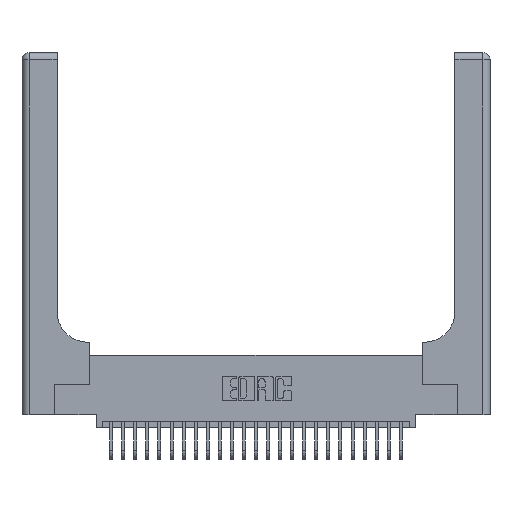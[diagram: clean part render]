
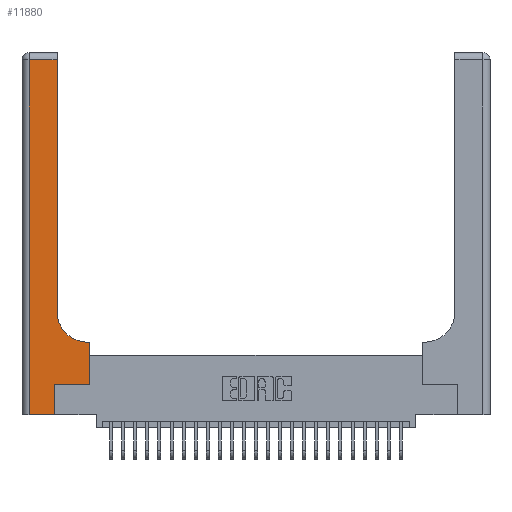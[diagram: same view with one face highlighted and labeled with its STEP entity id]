
A CAD part, top view. The second image highlights one B-rep face of the part: STEP entity #11880.
In plain terms, the highlighted planar face has unit normal (0, 0, 1).
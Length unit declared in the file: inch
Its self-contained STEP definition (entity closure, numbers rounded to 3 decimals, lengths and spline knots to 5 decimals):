
#184 = LINE ( 'NONE', #10783, #22507 ) ;
#234 = VERTEX_POINT ( 'NONE', #27878 ) ;
#263 = LINE ( 'NONE', #14552, #23274 ) ;
#578 = CARTESIAN_POINT ( 'NONE',  ( 0.2915, 2.94, 0.37 ) ) ;
#586 = LINE ( 'NONE', #12785, #11682 ) ;
#957 = VERTEX_POINT ( 'NONE', #14197 ) ;
#1566 = ORIENTED_EDGE ( 'NONE', *, *, #22909, .T. ) ;
#1987 = DIRECTION ( 'NONE',  ( -1., 0., 0. ) ) ;
#2071 = VECTOR ( 'NONE', #10237, 39.37008 ) ;
#2457 = EDGE_CURVE ( 'NONE', #8559, #4400, #23183, .T. ) ;
#3621 = ORIENTED_EDGE ( 'NONE', *, *, #8796, .T. ) ;
#3744 = ORIENTED_EDGE ( 'NONE', *, *, #2457, .T. ) ;
#4316 = EDGE_LOOP ( 'NONE', ( #9998, #3744, #8403, #5873, #7416, #1566, #3621, #21140, #25136 ) ) ;
#4400 = VERTEX_POINT ( 'NONE', #11769 ) ;
#5567 = CARTESIAN_POINT ( 'NONE',  ( 0.5415, 0.85, 0.37 ) ) ;
#5576 = CARTESIAN_POINT ( 'NONE',  ( 0.269, 0., 0.37 ) ) ;
#5873 = ORIENTED_EDGE ( 'NONE', *, *, #6956, .T. ) ;
#5915 = DIRECTION ( 'NONE',  ( 0., 1., 0. ) ) ;
#6107 = VECTOR ( 'NONE', #19537, 39.37008 ) ;
#6956 = EDGE_CURVE ( 'NONE', #22199, #957, #263, .T. ) ;
#7341 = DIRECTION ( 'NONE',  ( 0., 0., -1. ) ) ;
#7416 = ORIENTED_EDGE ( 'NONE', *, *, #25411, .T. ) ;
#7780 = DIRECTION ( 'NONE',  ( 1., 0., 0. ) ) ;
#7938 = DIRECTION ( 'NONE',  ( 1., 0., 0. ) ) ;
#8122 = CARTESIAN_POINT ( 'NONE',  ( 0., 2.94, 0.37 ) ) ;
#8403 = ORIENTED_EDGE ( 'NONE', *, *, #11023, .T. ) ;
#8559 = VERTEX_POINT ( 'NONE', #578 ) ;
#8796 = EDGE_CURVE ( 'NONE', #12746, #11222, #11831, .T. ) ;
#9263 = LINE ( 'NONE', #5576, #14498 ) ;
#9995 = DIRECTION ( 'NONE',  ( 0., 1., 0. ) ) ;
#9998 = ORIENTED_EDGE ( 'NONE', *, *, #26232, .T. ) ;
#10237 = DIRECTION ( 'NONE',  ( 1., 0., 0. ) ) ;
#10783 = CARTESIAN_POINT ( 'NONE',  ( 0.2915, 0.6, 0.37 ) ) ;
#11023 = EDGE_CURVE ( 'NONE', #4400, #22199, #586, .T. ) ;
#11222 = VERTEX_POINT ( 'NONE', #22989 ) ;
#11680 = PLANE ( 'NONE',  #18655 ) ;
#11682 = VECTOR ( 'NONE', #28460, 39.37008 ) ;
#11769 = CARTESIAN_POINT ( 'NONE',  ( 0.06, 2.94, 0.37 ) ) ;
#11831 = LINE ( 'NONE', #14741, #22335 ) ;
#11880 = ADVANCED_FACE ( 'NONE', ( #15141 ), #11680, .F. ) ;
#12746 = VERTEX_POINT ( 'NONE', #25901 ) ;
#12785 = CARTESIAN_POINT ( 'NONE',  ( 0.06, 3., 0.37 ) ) ;
#13308 = CARTESIAN_POINT ( 'NONE',  ( 0.06, 0., 0.37 ) ) ;
#14197 = CARTESIAN_POINT ( 'NONE',  ( 0.269, 0., 0.37 ) ) ;
#14228 = VERTEX_POINT ( 'NONE', #17385 ) ;
#14498 = VECTOR ( 'NONE', #9995, 39.37008 ) ;
#14552 = CARTESIAN_POINT ( 'NONE',  ( 0., 0., 0.37 ) ) ;
#14738 = CARTESIAN_POINT ( 'NONE',  ( 0.5415, 0.6, 0.37 ) ) ;
#14741 = CARTESIAN_POINT ( 'NONE',  ( 0.5585, 0.25, 0.37 ) ) ;
#15045 = CARTESIAN_POINT ( 'NONE',  ( 0.2915, 3., 0.37 ) ) ;
#15141 = FACE_OUTER_BOUND ( 'NONE', #4316, .T. ) ;
#15815 = VERTEX_POINT ( 'NONE', #14738 ) ;
#16176 = CARTESIAN_POINT ( 'NONE',  ( 0., 3., 0.37 ) ) ;
#17213 = VECTOR ( 'NONE', #19243, 39.37008 ) ;
#17385 = CARTESIAN_POINT ( 'NONE',  ( 0.2915, 0.85, 0.37 ) ) ;
#18655 = AXIS2_PLACEMENT_3D ( 'NONE', #16176, #7341, #22952 ) ;
#19243 = DIRECTION ( 'NONE',  ( -1., 0., 0. ) ) ;
#19537 = DIRECTION ( 'NONE',  ( 0., 1., 0. ) ) ;
#20847 = EDGE_CURVE ( 'NONE', #15815, #14228, #23133, .T. ) ;
#21140 = ORIENTED_EDGE ( 'NONE', *, *, #28042, .T. ) ;
#21148 = DIRECTION ( 'NONE',  ( 0., 0., -1. ) ) ;
#22199 = VERTEX_POINT ( 'NONE', #13308 ) ;
#22335 = VECTOR ( 'NONE', #5915, 39.37008 ) ;
#22507 = VECTOR ( 'NONE', #1987, 39.37008 ) ;
#22909 = EDGE_CURVE ( 'NONE', #234, #12746, #25107, .T. ) ;
#22952 = DIRECTION ( 'NONE',  ( -1., 0., 0. ) ) ;
#22989 = CARTESIAN_POINT ( 'NONE',  ( 0.5585, 0.6, 0.37 ) ) ;
#23133 = CIRCLE ( 'NONE', #23303, 0.25 ) ;
#23183 = LINE ( 'NONE', #8122, #17213 ) ;
#23197 = LINE ( 'NONE', #15045, #6107 ) ;
#23274 = VECTOR ( 'NONE', #7938, 39.37008 ) ;
#23303 = AXIS2_PLACEMENT_3D ( 'NONE', #5567, #21148, #7780 ) ;
#25107 = LINE ( 'NONE', #28159, #2071 ) ;
#25136 = ORIENTED_EDGE ( 'NONE', *, *, #20847, .T. ) ;
#25411 = EDGE_CURVE ( 'NONE', #957, #234, #9263, .T. ) ;
#25901 = CARTESIAN_POINT ( 'NONE',  ( 0.5585, 0.25, 0.37 ) ) ;
#26232 = EDGE_CURVE ( 'NONE', #14228, #8559, #23197, .T. ) ;
#27878 = CARTESIAN_POINT ( 'NONE',  ( 0.269, 0.25, 0.37 ) ) ;
#28042 = EDGE_CURVE ( 'NONE', #11222, #15815, #184, .T. ) ;
#28159 = CARTESIAN_POINT ( 'NONE',  ( 0.269, 0.25, 0.37 ) ) ;
#28460 = DIRECTION ( 'NONE',  ( 0., -1., 0. ) ) ;
